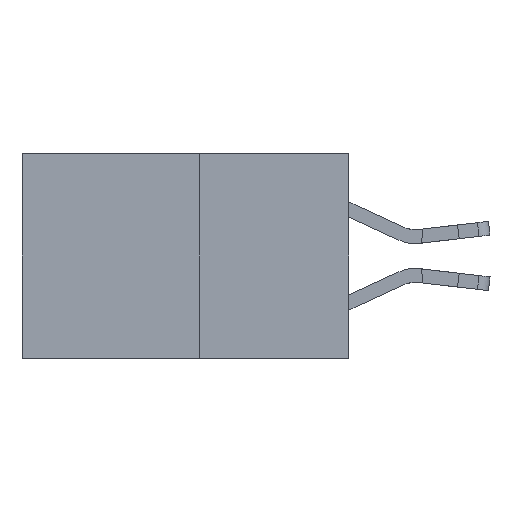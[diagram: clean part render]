
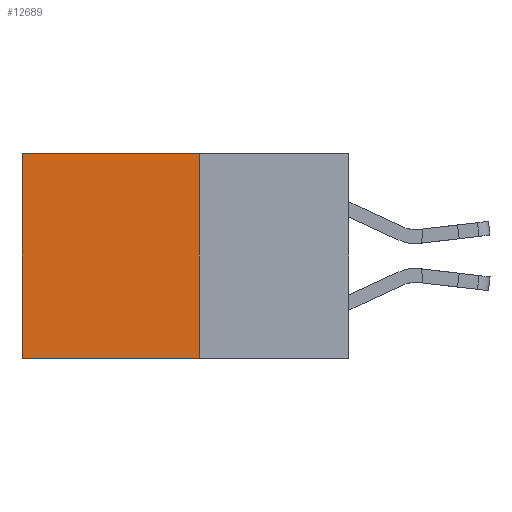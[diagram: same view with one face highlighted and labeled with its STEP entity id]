
A CAD part, left-side view. The second image highlights one B-rep face of the part: STEP entity #12689.
In plain terms, the highlighted planar face has unit normal (-1, 0, 0).
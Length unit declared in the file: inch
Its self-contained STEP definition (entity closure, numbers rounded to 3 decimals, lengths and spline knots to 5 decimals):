
#110 = ORIENTED_EDGE ( 'NONE', *, *, #4377, .F. ) ;
#648 = CARTESIAN_POINT ( 'NONE',  ( 0.277, 0.59, -0.37 ) ) ;
#1453 = CARTESIAN_POINT ( 'NONE',  ( 0.277, 0.27, -0.37 ) ) ;
#1638 = VECTOR ( 'NONE', #7303, 39.37008 ) ;
#2065 = ORIENTED_EDGE ( 'NONE', *, *, #12849, .F. ) ;
#2244 = VECTOR ( 'NONE', #8808, 39.37008 ) ;
#2564 = VERTEX_POINT ( 'NONE', #3657 ) ;
#2623 = DIRECTION ( 'NONE',  ( 0., 0., -1. ) ) ;
#3078 = CARTESIAN_POINT ( 'NONE',  ( 0.277, 0.27, -0.37 ) ) ;
#3657 = CARTESIAN_POINT ( 'NONE',  ( 0.277, 0.59, 0. ) ) ;
#4377 = EDGE_CURVE ( 'NONE', #10127, #10673, #7193, .T. ) ;
#4407 = FACE_OUTER_BOUND ( 'NONE', #5272, .T. ) ;
#4589 = ORIENTED_EDGE ( 'NONE', *, *, #8387, .T. ) ;
#5272 = EDGE_LOOP ( 'NONE', ( #6940, #2065, #110, #4589 ) ) ;
#6351 = DIRECTION ( 'NONE',  ( 0., 0., -1. ) ) ;
#6849 = VECTOR ( 'NONE', #6351, 39.37008 ) ;
#6940 = ORIENTED_EDGE ( 'NONE', *, *, #10137, .T. ) ;
#7193 = LINE ( 'NONE', #12967, #6849 ) ;
#7303 = DIRECTION ( 'NONE',  ( 0., 1., 0. ) ) ;
#8313 = PLANE ( 'NONE',  #9971 ) ;
#8387 = EDGE_CURVE ( 'NONE', #10127, #2564, #13581, .T. ) ;
#8445 = CARTESIAN_POINT ( 'NONE',  ( 0.277, 0.27, -0.37 ) ) ;
#8808 = DIRECTION ( 'NONE',  ( 0., 1., 0. ) ) ;
#9420 = DIRECTION ( 'NONE',  ( 1., 0., 0. ) ) ;
#9513 = VERTEX_POINT ( 'NONE', #10463 ) ;
#9971 = AXIS2_PLACEMENT_3D ( 'NONE', #1453, #9420, #2623 ) ;
#10127 = VERTEX_POINT ( 'NONE', #11905 ) ;
#10137 = EDGE_CURVE ( 'NONE', #2564, #9513, #14214, .T. ) ;
#10463 = CARTESIAN_POINT ( 'NONE',  ( 0.277, 0.59, -0.37 ) ) ;
#10673 = VERTEX_POINT ( 'NONE', #8445 ) ;
#11675 = CARTESIAN_POINT ( 'NONE',  ( 0.277, 0.27, 0. ) ) ;
#11854 = DIRECTION ( 'NONE',  ( 0., 0., -1. ) ) ;
#11905 = CARTESIAN_POINT ( 'NONE',  ( 0.277, 0.27, 0. ) ) ;
#12689 = ADVANCED_FACE ( 'NONE', ( #4407 ), #8313, .F. ) ;
#12849 = EDGE_CURVE ( 'NONE', #10673, #9513, #14157, .T. ) ;
#12967 = CARTESIAN_POINT ( 'NONE',  ( 0.277, 0.27, -0.37 ) ) ;
#13520 = VECTOR ( 'NONE', #11854, 39.37008 ) ;
#13581 = LINE ( 'NONE', #11675, #1638 ) ;
#14157 = LINE ( 'NONE', #3078, #2244 ) ;
#14214 = LINE ( 'NONE', #648, #13520 ) ;
